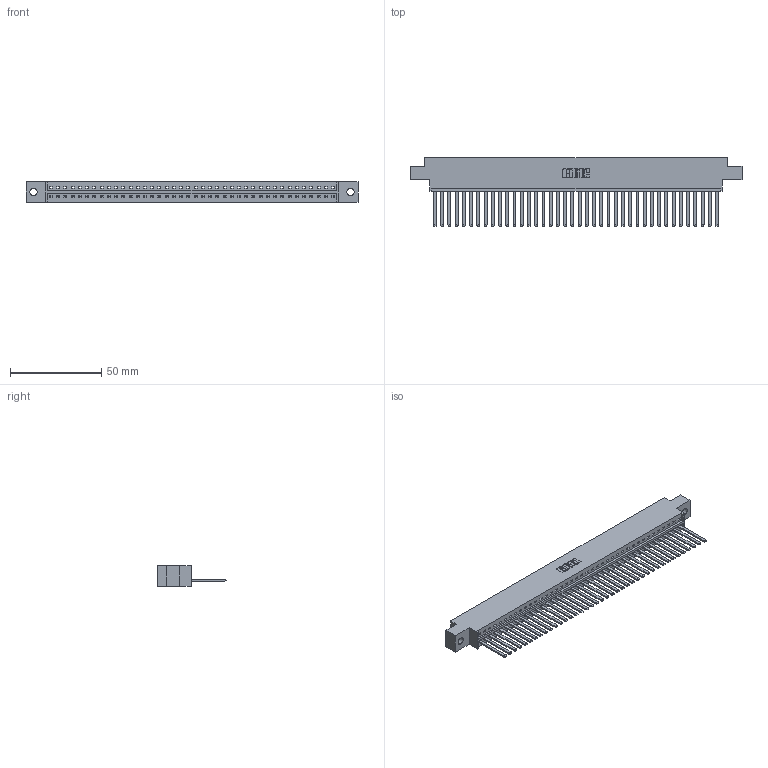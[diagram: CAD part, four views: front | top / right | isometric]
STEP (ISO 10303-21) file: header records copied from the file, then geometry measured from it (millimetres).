
FILE_DESCRIPTION (( 'STEP AP203' ), '1' );
FILE_NAME ('336-040-541-604.STEP', '2020-08-07T23:16:33', ( '' ), ( '' ), 'SwSTEP 2.0', 'SolidWorks 2020', '' );
FILE_SCHEMA (( 'CONFIG_CONTROL_DESIGN' ));
Length unit declared in the file: inch
Products named in the file (3): 336-040-541-604; 336-290-001_336-290-541; 336 Part_Offset - .156 Dia - TH
Assembly tree (41 placements, depth 2):
  336-040-541-604
    336 Part_Offset - .156 Dia - TH
    336-290-001_336-290-541  x40
Bounding box: 181.89 x 37.34 x 11.1 mm (x, y, z)
Volume: 26355.5 mm3; surface area: 28541.5 mm2
Topology: 41 solids, 41 shells, 2118 faces, 6483 edges, 4294 vertices
Faces by surface type: plane 1434, cylinder 684
Entity records: 29846 total; most frequent: CARTESIAN_POINT 5289, ORIENTED_EDGE 5166, DIRECTION 4359, EDGE_CURVE 2583, LINE 2451, VECTOR 2451, VERTEX_POINT 1720, AXIS2_PLACEMENT_3D 954
